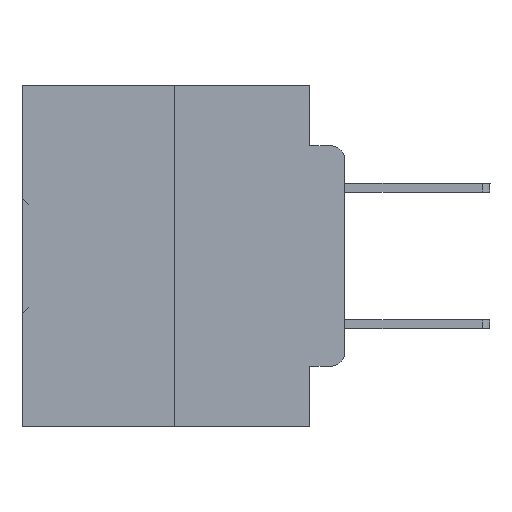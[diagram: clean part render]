
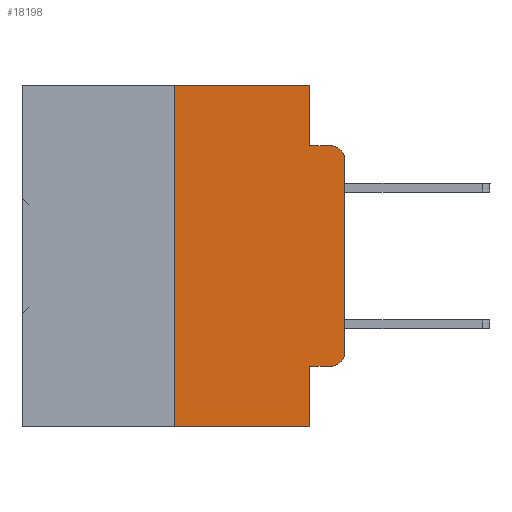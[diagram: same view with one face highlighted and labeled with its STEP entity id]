
A CAD part, left-side view. The second image highlights one B-rep face of the part: STEP entity #18198.
In plain terms, the highlighted planar face has unit normal (-1, 0, 0).
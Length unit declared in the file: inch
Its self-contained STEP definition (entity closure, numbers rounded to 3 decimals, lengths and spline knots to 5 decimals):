
#238 = LINE ( 'NONE', #26381, #19621 ) ;
#250 = DIRECTION ( 'NONE',  ( 0., 0., -1. ) ) ;
#272 = ORIENTED_EDGE ( 'NONE', *, *, #26610, .F. ) ;
#827 = EDGE_CURVE ( 'NONE', #7740, #16892, #35870, .T. ) ;
#859 = VECTOR ( 'NONE', #28374, 39.37008 ) ;
#1274 = ORIENTED_EDGE ( 'NONE', *, *, #11896, .F. ) ;
#1823 = CARTESIAN_POINT ( 'NONE',  ( 0., 0.051, -0.0885 ) ) ;
#2110 = DIRECTION ( 'NONE',  ( 0., 0., -1. ) ) ;
#2166 = CARTESIAN_POINT ( 'NONE',  ( 0., 0.051, -0.0885 ) ) ;
#3285 = CARTESIAN_POINT ( 'NONE',  ( 0., 0., -0.3915 ) ) ;
#4080 = CARTESIAN_POINT ( 'NONE',  ( 0., 0.473, 0. ) ) ;
#4235 = CARTESIAN_POINT ( 'NONE',  ( 0., 0., -0.1085 ) ) ;
#5418 = EDGE_CURVE ( 'NONE', #5926, #16892, #6684, .T. ) ;
#5926 = VERTEX_POINT ( 'NONE', #2166 ) ;
#6134 = FACE_OUTER_BOUND ( 'NONE', #13147, .T. ) ;
#6157 = ORIENTED_EDGE ( 'NONE', *, *, #14628, .T. ) ;
#6684 = LINE ( 'NONE', #1823, #19271 ) ;
#7591 = VERTEX_POINT ( 'NONE', #33080 ) ;
#7740 = VERTEX_POINT ( 'NONE', #4235 ) ;
#7845 = LINE ( 'NONE', #20066, #9201 ) ;
#8579 = ORIENTED_EDGE ( 'NONE', *, *, #12470, .T. ) ;
#8696 = VECTOR ( 'NONE', #16139, 39.37008 ) ;
#9201 = VECTOR ( 'NONE', #11236, 39.37008 ) ;
#10334 = CARTESIAN_POINT ( 'NONE',  ( 0., 0.051, 0. ) ) ;
#10366 = DIRECTION ( 'NONE',  ( -1., 0., 0. ) ) ;
#10541 = CARTESIAN_POINT ( 'NONE',  ( 0., 0.25, 0. ) ) ;
#10793 = CARTESIAN_POINT ( 'NONE',  ( 0., 0.02, -0.1085 ) ) ;
#11236 = DIRECTION ( 'NONE',  ( 0., 0., 1. ) ) ;
#11662 = LINE ( 'NONE', #4080, #26553 ) ;
#11896 = EDGE_CURVE ( 'NONE', #31748, #7591, #30225, .T. ) ;
#12470 = EDGE_CURVE ( 'NONE', #31748, #30588, #24776, .T. ) ;
#12740 = ORIENTED_EDGE ( 'NONE', *, *, #5418, .F. ) ;
#13147 = EDGE_LOOP ( 'NONE', ( #6157, #18734, #12740, #272, #23155, #32954, #15205, #1274, #8579, #19468 ) ) ;
#13900 = AXIS2_PLACEMENT_3D ( 'NONE', #33393, #16115, #24705 ) ;
#14628 = EDGE_CURVE ( 'NONE', #15316, #7740, #238, .T. ) ;
#15205 = ORIENTED_EDGE ( 'NONE', *, *, #36579, .T. ) ;
#15316 = VERTEX_POINT ( 'NONE', #3285 ) ;
#15909 = CARTESIAN_POINT ( 'NONE',  ( 0., 0.02, -0.3915 ) ) ;
#16115 = DIRECTION ( 'NONE',  ( 1., 0., 0. ) ) ;
#16139 = DIRECTION ( 'NONE',  ( 0., 0., -1. ) ) ;
#16192 = DIRECTION ( 'NONE',  ( 0., -1., 0. ) ) ;
#16892 = VERTEX_POINT ( 'NONE', #19443 ) ;
#18198 = ADVANCED_FACE ( 'NONE', ( #6134 ), #35776, .F. ) ;
#18579 = LINE ( 'NONE', #10334, #8696 ) ;
#18734 = ORIENTED_EDGE ( 'NONE', *, *, #827, .T. ) ;
#18991 = LINE ( 'NONE', #23737, #22150 ) ;
#19271 = VECTOR ( 'NONE', #16192, 39.37008 ) ;
#19443 = CARTESIAN_POINT ( 'NONE',  ( 0., 0.02, -0.0885 ) ) ;
#19468 = ORIENTED_EDGE ( 'NONE', *, *, #20081, .T. ) ;
#19621 = VECTOR ( 'NONE', #26263, 39.37008 ) ;
#19922 = CARTESIAN_POINT ( 'NONE',  ( 0., 0.051, -0.4115 ) ) ;
#20066 = CARTESIAN_POINT ( 'NONE',  ( 0., 0.25, 0. ) ) ;
#20081 = EDGE_CURVE ( 'NONE', #30588, #15316, #35771, .T. ) ;
#20805 = DIRECTION ( 'NONE',  ( 0., -1., 0. ) ) ;
#22141 = AXIS2_PLACEMENT_3D ( 'NONE', #15909, #10366, #25123 ) ;
#22150 = VECTOR ( 'NONE', #20805, 39.37008 ) ;
#22561 = VECTOR ( 'NONE', #250, 39.37008 ) ;
#22582 = EDGE_CURVE ( 'NONE', #34062, #25263, #11662, .T. ) ;
#23155 = ORIENTED_EDGE ( 'NONE', *, *, #22582, .F. ) ;
#23737 = CARTESIAN_POINT ( 'NONE',  ( 0., 0.473, -0.5 ) ) ;
#23864 = DIRECTION ( 'NONE',  ( 0., -1., 0. ) ) ;
#24705 = DIRECTION ( 'NONE',  ( 0., 0., -1. ) ) ;
#24776 = LINE ( 'NONE', #28501, #859 ) ;
#24951 = CARTESIAN_POINT ( 'NONE',  ( 0., 0.051, 0. ) ) ;
#25048 = DIRECTION ( 'NONE',  ( -1., 0., 0. ) ) ;
#25123 = DIRECTION ( 'NONE',  ( 0., 0., -1. ) ) ;
#25263 = VERTEX_POINT ( 'NONE', #24951 ) ;
#26263 = DIRECTION ( 'NONE',  ( 0., 0., 1. ) ) ;
#26381 = CARTESIAN_POINT ( 'NONE',  ( 0., 0., 0. ) ) ;
#26553 = VECTOR ( 'NONE', #23864, 39.37008 ) ;
#26610 = EDGE_CURVE ( 'NONE', #25263, #5926, #18579, .T. ) ;
#28119 = CARTESIAN_POINT ( 'NONE',  ( 0., 0.25, -0.5 ) ) ;
#28374 = DIRECTION ( 'NONE',  ( 0., -1., 0. ) ) ;
#28501 = CARTESIAN_POINT ( 'NONE',  ( 0., 0.051, -0.4115 ) ) ;
#30225 = LINE ( 'NONE', #34302, #22561 ) ;
#30588 = VERTEX_POINT ( 'NONE', #34075 ) ;
#31748 = VERTEX_POINT ( 'NONE', #19922 ) ;
#32954 = ORIENTED_EDGE ( 'NONE', *, *, #35102, .F. ) ;
#33080 = CARTESIAN_POINT ( 'NONE',  ( 0., 0.051, -0.5 ) ) ;
#33393 = CARTESIAN_POINT ( 'NONE',  ( 0., 0.473, 0. ) ) ;
#33465 = VERTEX_POINT ( 'NONE', #28119 ) ;
#33779 = AXIS2_PLACEMENT_3D ( 'NONE', #10793, #25048, #2110 ) ;
#34062 = VERTEX_POINT ( 'NONE', #10541 ) ;
#34075 = CARTESIAN_POINT ( 'NONE',  ( 0., 0.02, -0.4115 ) ) ;
#34302 = CARTESIAN_POINT ( 'NONE',  ( 0., 0.051, 0. ) ) ;
#35102 = EDGE_CURVE ( 'NONE', #33465, #34062, #7845, .T. ) ;
#35771 = CIRCLE ( 'NONE', #22141, 0.02 ) ;
#35776 = PLANE ( 'NONE',  #13900 ) ;
#35870 = CIRCLE ( 'NONE', #33779, 0.02 ) ;
#36579 = EDGE_CURVE ( 'NONE', #33465, #7591, #18991, .T. ) ;
